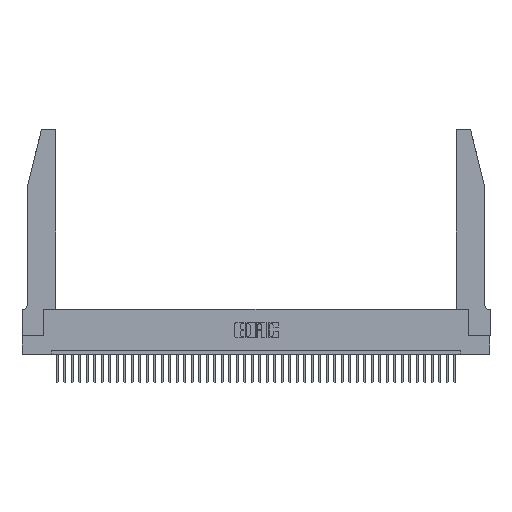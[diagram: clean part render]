
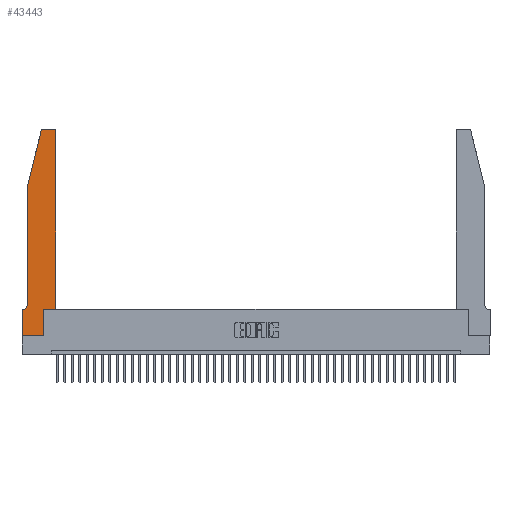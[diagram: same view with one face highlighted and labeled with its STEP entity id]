
A CAD part, top view. The second image highlights one B-rep face of the part: STEP entity #43443.
In plain terms, the highlighted planar face has unit normal (0, 0, 1).
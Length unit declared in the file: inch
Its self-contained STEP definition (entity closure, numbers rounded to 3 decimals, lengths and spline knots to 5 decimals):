
#211 = ORIENTED_EDGE ( 'NONE', *, *, #31523, .T. ) ;
#316 = DIRECTION ( 'NONE',  ( 0., 1., 0. ) ) ;
#619 = VECTOR ( 'NONE', #22521, 39.37008 ) ;
#885 = VERTEX_POINT ( 'NONE', #12914 ) ;
#1060 = ORIENTED_EDGE ( 'NONE', *, *, #42613, .T. ) ;
#1732 = VECTOR ( 'NONE', #41682, 39.37008 ) ;
#2002 = VECTOR ( 'NONE', #14170, 39.37008 ) ;
#2203 = VERTEX_POINT ( 'NONE', #2629 ) ;
#2629 = CARTESIAN_POINT ( 'NONE',  ( 0.25487, 2.72718, 0.37 ) ) ;
#3268 = VERTEX_POINT ( 'NONE', #12950 ) ;
#3768 = ORIENTED_EDGE ( 'NONE', *, *, #13871, .T. ) ;
#3797 = VERTEX_POINT ( 'NONE', #13652 ) ;
#3983 = LINE ( 'NONE', #28376, #33165 ) ;
#4721 = AXIS2_PLACEMENT_3D ( 'NONE', #31919, #24726, #8065 ) ;
#4931 = VERTEX_POINT ( 'NONE', #12566 ) ;
#5020 = VERTEX_POINT ( 'NONE', #10826 ) ;
#6516 = EDGE_CURVE ( 'NONE', #3268, #38916, #23469, .T. ) ;
#6692 = LINE ( 'NONE', #36796, #42183 ) ;
#6930 = PLANE ( 'NONE',  #7968 ) ;
#6997 = DIRECTION ( 'NONE',  ( 1., 0., 0. ) ) ;
#7240 = EDGE_CURVE ( 'NONE', #11486, #2203, #18014, .T. ) ;
#7363 = CARTESIAN_POINT ( 'NONE',  ( 0.4505, 0.35, 0.37 ) ) ;
#7598 = ORIENTED_EDGE ( 'NONE', *, *, #17372, .T. ) ;
#7864 = DIRECTION ( 'NONE',  ( -1., 0., 0. ) ) ;
#7968 = AXIS2_PLACEMENT_3D ( 'NONE', #10451, #24280, #10871 ) ;
#8065 = DIRECTION ( 'NONE',  ( -1., 0., 0. ) ) ;
#8798 = VERTEX_POINT ( 'NONE', #25220 ) ;
#9674 = FACE_OUTER_BOUND ( 'NONE', #31900, .T. ) ;
#10451 = CARTESIAN_POINT ( 'NONE',  ( 0., 0.35, 0.37 ) ) ;
#10617 = EDGE_CURVE ( 'NONE', #38916, #32477, #22571, .T. ) ;
#10826 = CARTESIAN_POINT ( 'NONE',  ( 0.2865, 0., 0.37 ) ) ;
#10871 = DIRECTION ( 'NONE',  ( 1., 0., 0. ) ) ;
#11486 = VERTEX_POINT ( 'NONE', #12699 ) ;
#12328 = DIRECTION ( 'NONE',  ( 1., 0., 0. ) ) ;
#12566 = CARTESIAN_POINT ( 'NONE',  ( 0., 0.35, 0.37 ) ) ;
#12699 = CARTESIAN_POINT ( 'NONE',  ( 0.284, 2.75, 0.37 ) ) ;
#12914 = CARTESIAN_POINT ( 'NONE',  ( 0.4505, 0.35, 0.37 ) ) ;
#12950 = CARTESIAN_POINT ( 'NONE',  ( 0.0755, 2., 0.37 ) ) ;
#13652 = CARTESIAN_POINT ( 'NONE',  ( 0.4205, 2.75, 0.37 ) ) ;
#13871 = EDGE_CURVE ( 'NONE', #3797, #11486, #31216, .T. ) ;
#14111 = LINE ( 'NONE', #7363, #2002 ) ;
#14170 = DIRECTION ( 'NONE',  ( 1., 0., 0. ) ) ;
#14576 = CARTESIAN_POINT ( 'NONE',  ( 0., 0., 0.37 ) ) ;
#14838 = CIRCLE ( 'NONE', #32654, 0.03 ) ;
#15399 = CARTESIAN_POINT ( 'NONE',  ( 0.284, 2.72, 0.37 ) ) ;
#16530 = DIRECTION ( 'NONE',  ( 0., 1., 0. ) ) ;
#16671 = VERTEX_POINT ( 'NONE', #25572 ) ;
#17185 = CARTESIAN_POINT ( 'NONE',  ( 0.2865, 0.35, 0.37 ) ) ;
#17372 = EDGE_CURVE ( 'NONE', #4931, #34118, #28756, .T. ) ;
#18014 = CIRCLE ( 'NONE', #30465, 0.03 ) ;
#18169 = ORIENTED_EDGE ( 'NONE', *, *, #10617, .T. ) ;
#19800 = DIRECTION ( 'NONE',  ( -0.239, -0.971, 0. ) ) ;
#19882 = CARTESIAN_POINT ( 'NONE',  ( 0.0755, 0.42, 0.37 ) ) ;
#20112 = ORIENTED_EDGE ( 'NONE', *, *, #36738, .T. ) ;
#20746 = EDGE_CURVE ( 'NONE', #8798, #885, #14111, .T. ) ;
#21300 = CARTESIAN_POINT ( 'NONE',  ( 0.0755, 0.35, 0.37 ) ) ;
#21420 = EDGE_CURVE ( 'NONE', #34118, #5020, #3983, .T. ) ;
#22521 = DIRECTION ( 'NONE',  ( 0., -1., 0. ) ) ;
#22571 = CIRCLE ( 'NONE', #4721, 0.07 ) ;
#22831 = VECTOR ( 'NONE', #38490, 39.37008 ) ;
#23469 = LINE ( 'NONE', #42721, #619 ) ;
#24280 = DIRECTION ( 'NONE',  ( 0., 0., 1. ) ) ;
#24542 = DIRECTION ( 'NONE',  ( 1., 0., 0. ) ) ;
#24726 = DIRECTION ( 'NONE',  ( 0., 0., -1. ) ) ;
#24891 = ORIENTED_EDGE ( 'NONE', *, *, #21420, .T. ) ;
#25220 = CARTESIAN_POINT ( 'NONE',  ( 0.2865, 0.35, 0.37 ) ) ;
#25572 = CARTESIAN_POINT ( 'NONE',  ( 0.4505, 2.72, 0.37 ) ) ;
#27299 = ORIENTED_EDGE ( 'NONE', *, *, #7240, .T. ) ;
#27494 = ORIENTED_EDGE ( 'NONE', *, *, #29825, .T. ) ;
#27623 = DIRECTION ( 'NONE',  ( 0., 0., 1. ) ) ;
#27889 = CARTESIAN_POINT ( 'NONE',  ( 0.4205, 2.72, 0.37 ) ) ;
#28376 = CARTESIAN_POINT ( 'NONE',  ( 0., 0., 0.37 ) ) ;
#28756 = LINE ( 'NONE', #14576, #1732 ) ;
#29591 = LINE ( 'NONE', #21300, #40655 ) ;
#29825 = EDGE_CURVE ( 'NONE', #16671, #3797, #14838, .T. ) ;
#30110 = CARTESIAN_POINT ( 'NONE',  ( 0.0755, 2., 0.37 ) ) ;
#30465 = AXIS2_PLACEMENT_3D ( 'NONE', #15399, #39225, #12328 ) ;
#31216 = LINE ( 'NONE', #38802, #22831 ) ;
#31330 = VECTOR ( 'NONE', #316, 39.37008 ) ;
#31523 = EDGE_CURVE ( 'NONE', #32477, #4931, #29591, .T. ) ;
#31900 = EDGE_LOOP ( 'NONE', ( #3768, #27299, #1060, #43270, #18169, #211, #7598, #24891, #20112, #37994, #39794, #27494 ) ) ;
#31919 = CARTESIAN_POINT ( 'NONE',  ( 0.0055, 0.42, 0.37 ) ) ;
#32477 = VERTEX_POINT ( 'NONE', #36597 ) ;
#32654 = AXIS2_PLACEMENT_3D ( 'NONE', #27889, #27623, #6997 ) ;
#33165 = VECTOR ( 'NONE', #24542, 39.37008 ) ;
#34118 = VERTEX_POINT ( 'NONE', #39109 ) ;
#34517 = LINE ( 'NONE', #17185, #31330 ) ;
#36597 = CARTESIAN_POINT ( 'NONE',  ( 0.0055, 0.35, 0.37 ) ) ;
#36738 = EDGE_CURVE ( 'NONE', #5020, #8798, #34517, .T. ) ;
#36796 = CARTESIAN_POINT ( 'NONE',  ( 0.4505, 0.35, 0.37 ) ) ;
#37994 = ORIENTED_EDGE ( 'NONE', *, *, #20746, .T. ) ;
#38490 = DIRECTION ( 'NONE',  ( -1., 0., 0. ) ) ;
#38802 = CARTESIAN_POINT ( 'NONE',  ( 0.2605, 2.75, 0.37 ) ) ;
#38916 = VERTEX_POINT ( 'NONE', #19882 ) ;
#39109 = CARTESIAN_POINT ( 'NONE',  ( 0., 0., 0.37 ) ) ;
#39225 = DIRECTION ( 'NONE',  ( 0., 0., 1. ) ) ;
#39644 = EDGE_CURVE ( 'NONE', #885, #16671, #6692, .T. ) ;
#39794 = ORIENTED_EDGE ( 'NONE', *, *, #39644, .T. ) ;
#39955 = LINE ( 'NONE', #30110, #41483 ) ;
#40655 = VECTOR ( 'NONE', #7864, 39.37008 ) ;
#41483 = VECTOR ( 'NONE', #19800, 39.37008 ) ;
#41682 = DIRECTION ( 'NONE',  ( 0., -1., 0. ) ) ;
#42183 = VECTOR ( 'NONE', #16530, 39.37008 ) ;
#42613 = EDGE_CURVE ( 'NONE', #2203, #3268, #39955, .T. ) ;
#42721 = CARTESIAN_POINT ( 'NONE',  ( 0.0755, 2., 0.37 ) ) ;
#43270 = ORIENTED_EDGE ( 'NONE', *, *, #6516, .T. ) ;
#43443 = ADVANCED_FACE ( 'NONE', ( #9674 ), #6930, .T. ) ;
